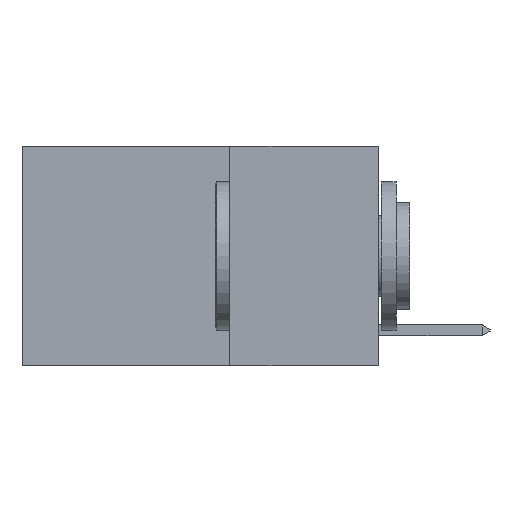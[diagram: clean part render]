
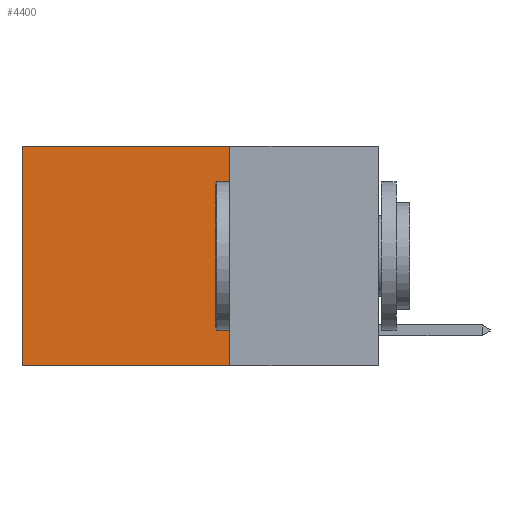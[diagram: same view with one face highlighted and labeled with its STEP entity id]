
A CAD part, left-side view. The second image highlights one B-rep face of the part: STEP entity #4400.
In plain terms, the highlighted planar face has unit normal (-1, 0, 0).
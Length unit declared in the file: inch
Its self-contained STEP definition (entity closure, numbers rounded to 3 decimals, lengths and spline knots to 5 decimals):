
#73 = DIRECTION ( 'NONE',  ( 0., 0., -1. ) ) ;
#91 = DIRECTION ( 'NONE',  ( 1., 0., 0. ) ) ;
#124 = PLANE ( 'NONE',  #1114 ) ;
#161 = LINE ( 'NONE', #3469, #3854 ) ;
#184 = LINE ( 'NONE', #1090, #7650 ) ;
#346 = CARTESIAN_POINT ( 'NONE',  ( 0.2625, 0.25, 0. ) ) ;
#532 = LINE ( 'NONE', #9042, #4442 ) ;
#619 = CARTESIAN_POINT ( 'NONE',  ( 0.2625, 0.6, -0.37 ) ) ;
#1090 = CARTESIAN_POINT ( 'NONE',  ( 0.2625, 0.6, 0. ) ) ;
#1114 = AXIS2_PLACEMENT_3D ( 'NONE', #346, #91, #73 ) ;
#1477 = VECTOR ( 'NONE', #7500, 39.37008 ) ;
#1518 = EDGE_CURVE ( 'NONE', #6460, #7272, #5773, .T. ) ;
#1732 = VERTEX_POINT ( 'NONE', #619 ) ;
#2757 = ORIENTED_EDGE ( 'NONE', *, *, #5819, .F. ) ;
#3469 = CARTESIAN_POINT ( 'NONE',  ( 0.2625, 0.25, 0. ) ) ;
#3514 = FACE_OUTER_BOUND ( 'NONE', #5921, .T. ) ;
#3854 = VECTOR ( 'NONE', #9154, 39.37008 ) ;
#3992 = ORIENTED_EDGE ( 'NONE', *, *, #1518, .F. ) ;
#4400 = ADVANCED_FACE ( 'NONE', ( #3514 ), #124, .F. ) ;
#4442 = VECTOR ( 'NONE', #5472, 39.37008 ) ;
#5176 = EDGE_CURVE ( 'NONE', #7731, #1732, #184, .T. ) ;
#5452 = DIRECTION ( 'NONE',  ( 0., 0., -1. ) ) ;
#5472 = DIRECTION ( 'NONE',  ( 0., 1., 0. ) ) ;
#5626 = ORIENTED_EDGE ( 'NONE', *, *, #6543, .T. ) ;
#5773 = LINE ( 'NONE', #6596, #1477 ) ;
#5819 = EDGE_CURVE ( 'NONE', #7272, #1732, #532, .T. ) ;
#5921 = EDGE_LOOP ( 'NONE', ( #7433, #2757, #3992, #5626 ) ) ;
#6283 = CARTESIAN_POINT ( 'NONE',  ( 0.2625, 0.6, 0. ) ) ;
#6460 = VERTEX_POINT ( 'NONE', #6860 ) ;
#6543 = EDGE_CURVE ( 'NONE', #6460, #7731, #161, .T. ) ;
#6596 = CARTESIAN_POINT ( 'NONE',  ( 0.2625, 0.25, 0. ) ) ;
#6860 = CARTESIAN_POINT ( 'NONE',  ( 0.2625, 0.25, 0. ) ) ;
#7272 = VERTEX_POINT ( 'NONE', #8624 ) ;
#7433 = ORIENTED_EDGE ( 'NONE', *, *, #5176, .T. ) ;
#7500 = DIRECTION ( 'NONE',  ( 0., 0., -1. ) ) ;
#7650 = VECTOR ( 'NONE', #5452, 39.37008 ) ;
#7731 = VERTEX_POINT ( 'NONE', #6283 ) ;
#8624 = CARTESIAN_POINT ( 'NONE',  ( 0.2625, 0.25, -0.37 ) ) ;
#9042 = CARTESIAN_POINT ( 'NONE',  ( 0.2625, 0.25, -0.37 ) ) ;
#9154 = DIRECTION ( 'NONE',  ( 0., 1., 0. ) ) ;
